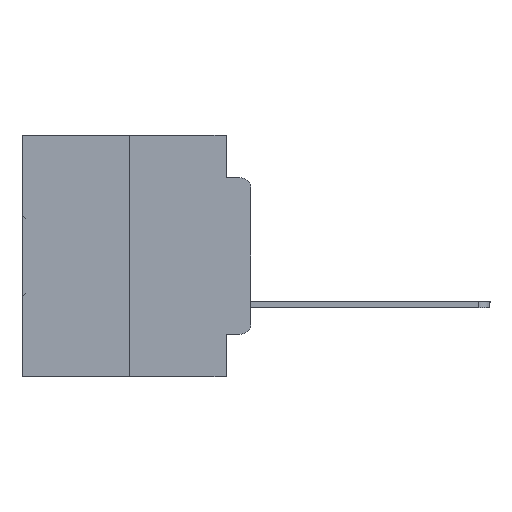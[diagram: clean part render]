
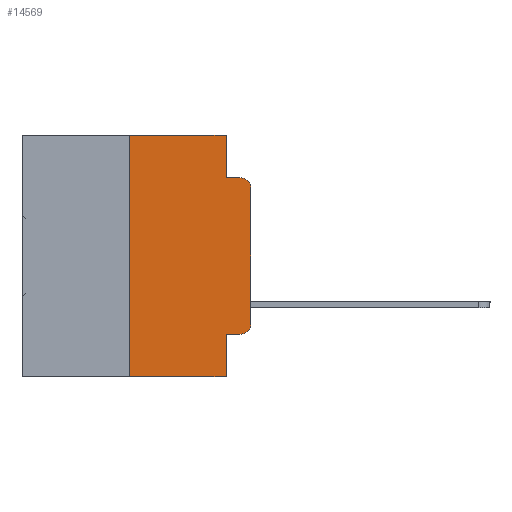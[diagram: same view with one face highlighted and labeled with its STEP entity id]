
A CAD part, left-side view. The second image highlights one B-rep face of the part: STEP entity #14569.
In plain terms, the highlighted planar face has unit normal (-1, 0, 0).
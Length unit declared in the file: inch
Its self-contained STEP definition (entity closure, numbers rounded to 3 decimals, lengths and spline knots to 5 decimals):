
#105 = EDGE_CURVE ( 'NONE', #1049, #31240, #21552, .T. ) ;
#203 = DIRECTION ( 'NONE',  ( 0., 0., -1. ) ) ;
#296 = EDGE_CURVE ( 'NONE', #28127, #25949, #26271, .T. ) ;
#699 = VECTOR ( 'NONE', #8848, 39.37008 ) ;
#1030 = CARTESIAN_POINT ( 'NONE',  ( 0., 0.25, -0.5 ) ) ;
#1049 = VERTEX_POINT ( 'NONE', #7410 ) ;
#1889 = CARTESIAN_POINT ( 'NONE',  ( 0., 0., -0.1085 ) ) ;
#1997 = ORIENTED_EDGE ( 'NONE', *, *, #33096, .T. ) ;
#2030 = EDGE_CURVE ( 'NONE', #31240, #12795, #25066, .T. ) ;
#2580 = VERTEX_POINT ( 'NONE', #18055 ) ;
#2931 = ORIENTED_EDGE ( 'NONE', *, *, #105, .F. ) ;
#3045 = CARTESIAN_POINT ( 'NONE',  ( 0., 0.051, 0. ) ) ;
#3593 = CARTESIAN_POINT ( 'NONE',  ( 0., 0.051, 0. ) ) ;
#3843 = CARTESIAN_POINT ( 'NONE',  ( 0., 0.051, -0.4115 ) ) ;
#3872 = AXIS2_PLACEMENT_3D ( 'NONE', #30878, #20068, #10226 ) ;
#5543 = VERTEX_POINT ( 'NONE', #31975 ) ;
#5585 = VECTOR ( 'NONE', #203, 39.37008 ) ;
#5756 = EDGE_CURVE ( 'NONE', #30290, #10887, #22835, .T. ) ;
#6211 = CARTESIAN_POINT ( 'NONE',  ( 0., 0.051, -0.0885 ) ) ;
#6486 = PLANE ( 'NONE',  #16600 ) ;
#6663 = EDGE_CURVE ( 'NONE', #13461, #12795, #28143, .T. ) ;
#7410 = CARTESIAN_POINT ( 'NONE',  ( 0., 0.051, 0. ) ) ;
#8207 = EDGE_CURVE ( 'NONE', #28127, #2580, #26888, .T. ) ;
#8377 = CARTESIAN_POINT ( 'NONE',  ( 0., 0.051, -0.5 ) ) ;
#8430 = CARTESIAN_POINT ( 'NONE',  ( 0., 0.051, -0.4115 ) ) ;
#8848 = DIRECTION ( 'NONE',  ( 0., -1., 0. ) ) ;
#9028 = DIRECTION ( 'NONE',  ( 0., 0., 1. ) ) ;
#10226 = DIRECTION ( 'NONE',  ( 0., 0., -1. ) ) ;
#10887 = VERTEX_POINT ( 'NONE', #19681 ) ;
#11384 = LINE ( 'NONE', #21719, #699 ) ;
#11408 = DIRECTION ( 'NONE',  ( 0., 0., -1. ) ) ;
#11578 = FACE_OUTER_BOUND ( 'NONE', #21740, .T. ) ;
#11837 = ORIENTED_EDGE ( 'NONE', *, *, #296, .F. ) ;
#12681 = DIRECTION ( 'NONE',  ( 0., -1., 0. ) ) ;
#12795 = VERTEX_POINT ( 'NONE', #28594 ) ;
#13461 = VERTEX_POINT ( 'NONE', #1889 ) ;
#14008 = ORIENTED_EDGE ( 'NONE', *, *, #6663, .T. ) ;
#14287 = LINE ( 'NONE', #24280, #19367 ) ;
#14569 = ADVANCED_FACE ( 'NONE', ( #11578 ), #6486, .F. ) ;
#14973 = VECTOR ( 'NONE', #18766, 39.37008 ) ;
#16286 = CIRCLE ( 'NONE', #3872, 0.02 ) ;
#16308 = VECTOR ( 'NONE', #12681, 39.37008 ) ;
#16365 = VECTOR ( 'NONE', #11408, 39.37008 ) ;
#16600 = AXIS2_PLACEMENT_3D ( 'NONE', #27314, #24618, #22243 ) ;
#17370 = ORIENTED_EDGE ( 'NONE', *, *, #28492, .T. ) ;
#17447 = CARTESIAN_POINT ( 'NONE',  ( 0., 0.02, -0.1085 ) ) ;
#17600 = ORIENTED_EDGE ( 'NONE', *, *, #5756, .F. ) ;
#17746 = CARTESIAN_POINT ( 'NONE',  ( 0., 0.051, -0.0885 ) ) ;
#18055 = CARTESIAN_POINT ( 'NONE',  ( 0., 0.02, -0.4115 ) ) ;
#18709 = ORIENTED_EDGE ( 'NONE', *, *, #25224, .F. ) ;
#18766 = DIRECTION ( 'NONE',  ( 0., -1., 0. ) ) ;
#19367 = VECTOR ( 'NONE', #9028, 39.37008 ) ;
#19681 = CARTESIAN_POINT ( 'NONE',  ( 0., 0.25, 0. ) ) ;
#20068 = DIRECTION ( 'NONE',  ( -1., 0., 0. ) ) ;
#21552 = LINE ( 'NONE', #3593, #16365 ) ;
#21719 = CARTESIAN_POINT ( 'NONE',  ( 0., 0.473, -0.5 ) ) ;
#21740 = EDGE_LOOP ( 'NONE', ( #17370, #14008, #28220, #2931, #18709, #17600, #33328, #11837, #23206, #1997 ) ) ;
#22151 = CARTESIAN_POINT ( 'NONE',  ( 0., 0.25, 0. ) ) ;
#22243 = DIRECTION ( 'NONE',  ( 0., 0., -1. ) ) ;
#22835 = LINE ( 'NONE', #22151, #30220 ) ;
#23206 = ORIENTED_EDGE ( 'NONE', *, *, #8207, .T. ) ;
#24280 = CARTESIAN_POINT ( 'NONE',  ( 0., 0., 0. ) ) ;
#24618 = DIRECTION ( 'NONE',  ( 1., 0., 0. ) ) ;
#24708 = DIRECTION ( 'NONE',  ( 0., -1., 0. ) ) ;
#24744 = EDGE_CURVE ( 'NONE', #30290, #25949, #11384, .T. ) ;
#25066 = LINE ( 'NONE', #17746, #16308 ) ;
#25224 = EDGE_CURVE ( 'NONE', #10887, #1049, #29778, .T. ) ;
#25949 = VERTEX_POINT ( 'NONE', #8377 ) ;
#26271 = LINE ( 'NONE', #3045, #5585 ) ;
#26888 = LINE ( 'NONE', #8430, #14973 ) ;
#26982 = VECTOR ( 'NONE', #24708, 39.37008 ) ;
#27314 = CARTESIAN_POINT ( 'NONE',  ( 0., 0.473, 0. ) ) ;
#27423 = DIRECTION ( 'NONE',  ( 0., 0., -1. ) ) ;
#28127 = VERTEX_POINT ( 'NONE', #3843 ) ;
#28143 = CIRCLE ( 'NONE', #30280, 0.02 ) ;
#28220 = ORIENTED_EDGE ( 'NONE', *, *, #2030, .F. ) ;
#28492 = EDGE_CURVE ( 'NONE', #5543, #13461, #14287, .T. ) ;
#28594 = CARTESIAN_POINT ( 'NONE',  ( 0., 0.02, -0.0885 ) ) ;
#29778 = LINE ( 'NONE', #33172, #26982 ) ;
#30220 = VECTOR ( 'NONE', #33156, 39.37008 ) ;
#30280 = AXIS2_PLACEMENT_3D ( 'NONE', #17447, #30620, #27423 ) ;
#30290 = VERTEX_POINT ( 'NONE', #1030 ) ;
#30620 = DIRECTION ( 'NONE',  ( -1., 0., 0. ) ) ;
#30878 = CARTESIAN_POINT ( 'NONE',  ( 0., 0.02, -0.3915 ) ) ;
#31240 = VERTEX_POINT ( 'NONE', #6211 ) ;
#31975 = CARTESIAN_POINT ( 'NONE',  ( 0., 0., -0.3915 ) ) ;
#33096 = EDGE_CURVE ( 'NONE', #2580, #5543, #16286, .T. ) ;
#33156 = DIRECTION ( 'NONE',  ( 0., 0., 1. ) ) ;
#33172 = CARTESIAN_POINT ( 'NONE',  ( 0., 0.473, 0. ) ) ;
#33328 = ORIENTED_EDGE ( 'NONE', *, *, #24744, .T. ) ;
